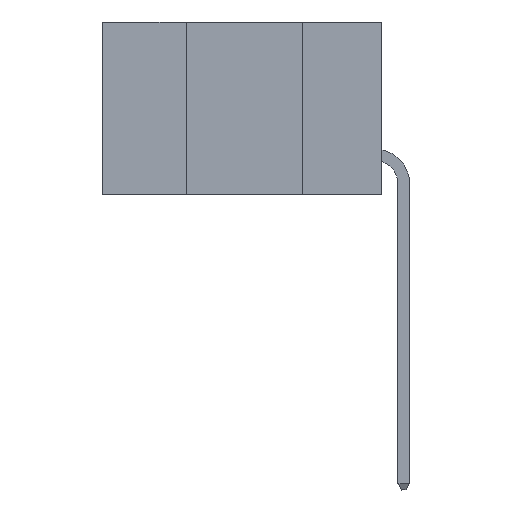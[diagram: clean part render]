
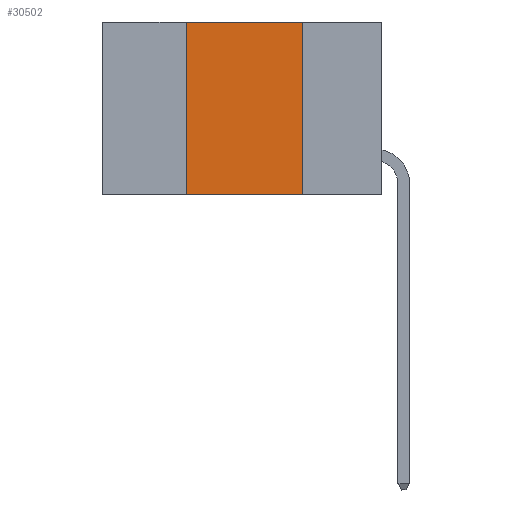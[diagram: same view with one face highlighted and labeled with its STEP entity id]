
A CAD part, left-side view. The second image highlights one B-rep face of the part: STEP entity #30502.
In plain terms, the highlighted planar face has unit normal (-1, 0, 0).
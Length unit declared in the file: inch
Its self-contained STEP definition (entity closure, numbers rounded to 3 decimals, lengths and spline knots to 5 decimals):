
#211 = DIRECTION ( 'NONE',  ( 0., 0., -1. ) ) ;
#953 = LINE ( 'NONE', #16945, #29306 ) ;
#2012 = LINE ( 'NONE', #6185, #36436 ) ;
#5009 = LINE ( 'NONE', #11564, #38993 ) ;
#6185 = CARTESIAN_POINT ( 'NONE',  ( 0., 0.6, 0. ) ) ;
#6836 = ORIENTED_EDGE ( 'NONE', *, *, #13099, .T. ) ;
#9666 = DIRECTION ( 'NONE',  ( 0., -1., 0. ) ) ;
#10961 = VERTEX_POINT ( 'NONE', #39072 ) ;
#11353 = VERTEX_POINT ( 'NONE', #42054 ) ;
#11564 = CARTESIAN_POINT ( 'NONE',  ( 0., 0.42, 0. ) ) ;
#12692 = ORIENTED_EDGE ( 'NONE', *, *, #19938, .F. ) ;
#13099 = EDGE_CURVE ( 'NONE', #11353, #22926, #953, .T. ) ;
#14781 = AXIS2_PLACEMENT_3D ( 'NONE', #17935, #32212, #211 ) ;
#16460 = CARTESIAN_POINT ( 'NONE',  ( 0., 0.17, 0. ) ) ;
#16945 = CARTESIAN_POINT ( 'NONE',  ( 0., 0.6, -0.37 ) ) ;
#17240 = DIRECTION ( 'NONE',  ( 0., -1., 0. ) ) ;
#17935 = CARTESIAN_POINT ( 'NONE',  ( 0., 0.6, 0. ) ) ;
#19924 = ORIENTED_EDGE ( 'NONE', *, *, #29688, .F. ) ;
#19938 = EDGE_CURVE ( 'NONE', #34610, #22926, #32084, .T. ) ;
#20495 = CARTESIAN_POINT ( 'NONE',  ( 0., 0.17, -0.37 ) ) ;
#22112 = VECTOR ( 'NONE', #26779, 39.37008 ) ;
#22594 = CARTESIAN_POINT ( 'NONE',  ( 0., 0.17, 0. ) ) ;
#22926 = VERTEX_POINT ( 'NONE', #20495 ) ;
#26779 = DIRECTION ( 'NONE',  ( 0., 0., -1. ) ) ;
#29110 = PLANE ( 'NONE',  #14781 ) ;
#29306 = VECTOR ( 'NONE', #9666, 39.37008 ) ;
#29688 = EDGE_CURVE ( 'NONE', #11353, #10961, #5009, .T. ) ;
#30502 = ADVANCED_FACE ( 'NONE', ( #34453 ), #29110, .F. ) ;
#32084 = LINE ( 'NONE', #22594, #22112 ) ;
#32212 = DIRECTION ( 'NONE',  ( 1., 0., 0. ) ) ;
#34453 = FACE_OUTER_BOUND ( 'NONE', #35499, .T. ) ;
#34610 = VERTEX_POINT ( 'NONE', #16460 ) ;
#35499 = EDGE_LOOP ( 'NONE', ( #12692, #38970, #19924, #6836 ) ) ;
#36436 = VECTOR ( 'NONE', #17240, 39.37008 ) ;
#38970 = ORIENTED_EDGE ( 'NONE', *, *, #43046, .F. ) ;
#38993 = VECTOR ( 'NONE', #43917, 39.37008 ) ;
#39072 = CARTESIAN_POINT ( 'NONE',  ( 0., 0.42, 0. ) ) ;
#42054 = CARTESIAN_POINT ( 'NONE',  ( 0., 0.42, -0.37 ) ) ;
#43046 = EDGE_CURVE ( 'NONE', #10961, #34610, #2012, .T. ) ;
#43917 = DIRECTION ( 'NONE',  ( 0., 0., 1. ) ) ;
